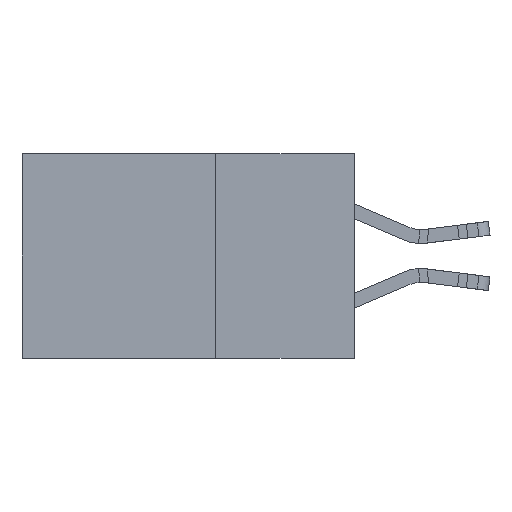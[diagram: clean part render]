
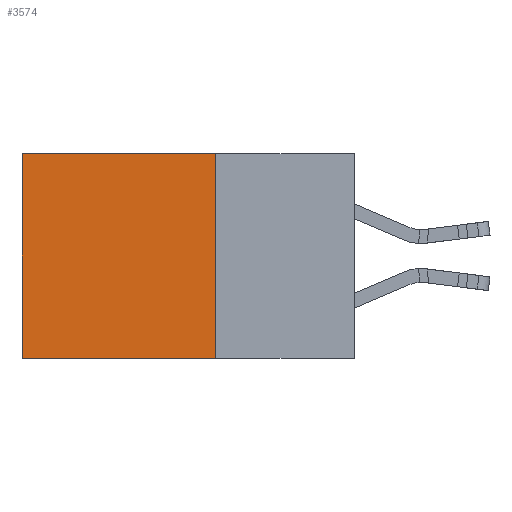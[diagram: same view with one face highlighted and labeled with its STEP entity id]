
A CAD part, left-side view. The second image highlights one B-rep face of the part: STEP entity #3574.
In plain terms, the highlighted planar face has unit normal (-1, 0, 0).
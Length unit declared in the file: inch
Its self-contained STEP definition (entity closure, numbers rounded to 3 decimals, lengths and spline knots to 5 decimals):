
#2606 = DIRECTION ( 'NONE',  ( 0., 0., -1. ) ) ;
#2619 = EDGE_CURVE ( 'NONE', #5461, #28859, #26973, .T. ) ;
#3574 = ADVANCED_FACE ( 'NONE', ( #20780 ), #10908, .F. ) ;
#4157 = ORIENTED_EDGE ( 'NONE', *, *, #2619, .T. ) ;
#5461 = VERTEX_POINT ( 'NONE', #24107 ) ;
#6086 = AXIS2_PLACEMENT_3D ( 'NONE', #10902, #10879, #10489 ) ;
#8408 = CARTESIAN_POINT ( 'NONE',  ( 0.298, 0.25, -0.37 ) ) ;
#8775 = EDGE_LOOP ( 'NONE', ( #9662, #10339, #9751, #4157 ) ) ;
#8953 = CARTESIAN_POINT ( 'NONE',  ( 0.298, 0.6, 0. ) ) ;
#8996 = VERTEX_POINT ( 'NONE', #25405 ) ;
#9223 = VECTOR ( 'NONE', #15777, 39.37008 ) ;
#9247 = VECTOR ( 'NONE', #11238, 39.37008 ) ;
#9662 = ORIENTED_EDGE ( 'NONE', *, *, #21631, .T. ) ;
#9751 = ORIENTED_EDGE ( 'NONE', *, *, #11562, .F. ) ;
#10339 = ORIENTED_EDGE ( 'NONE', *, *, #26287, .F. ) ;
#10489 = DIRECTION ( 'NONE',  ( 0., 0., -1. ) ) ;
#10684 = DIRECTION ( 'NONE',  ( 0., 1., 0. ) ) ;
#10879 = DIRECTION ( 'NONE',  ( 1., 0., 0. ) ) ;
#10902 = CARTESIAN_POINT ( 'NONE',  ( 0.298, 0.25, 0. ) ) ;
#10908 = PLANE ( 'NONE',  #6086 ) ;
#11147 = VECTOR ( 'NONE', #10684, 39.37008 ) ;
#11238 = DIRECTION ( 'NONE',  ( 0., 0., -1. ) ) ;
#11562 = EDGE_CURVE ( 'NONE', #5461, #23902, #22540, .T. ) ;
#12257 = CARTESIAN_POINT ( 'NONE',  ( 0.298, 0.25, 0. ) ) ;
#13918 = CARTESIAN_POINT ( 'NONE',  ( 0.298, 0.25, 0. ) ) ;
#15777 = DIRECTION ( 'NONE',  ( 0., 1., 0. ) ) ;
#20780 = FACE_OUTER_BOUND ( 'NONE', #8775, .T. ) ;
#21631 = EDGE_CURVE ( 'NONE', #28859, #8996, #26994, .T. ) ;
#22540 = LINE ( 'NONE', #13918, #27623 ) ;
#23902 = VERTEX_POINT ( 'NONE', #28627 ) ;
#24107 = CARTESIAN_POINT ( 'NONE',  ( 0.298, 0.25, 0. ) ) ;
#25405 = CARTESIAN_POINT ( 'NONE',  ( 0.298, 0.6, -0.37 ) ) ;
#26287 = EDGE_CURVE ( 'NONE', #23902, #8996, #28810, .T. ) ;
#26973 = LINE ( 'NONE', #12257, #9223 ) ;
#26994 = LINE ( 'NONE', #8953, #9247 ) ;
#27623 = VECTOR ( 'NONE', #2606, 39.37008 ) ;
#28456 = CARTESIAN_POINT ( 'NONE',  ( 0.298, 0.6, 0. ) ) ;
#28627 = CARTESIAN_POINT ( 'NONE',  ( 0.298, 0.25, -0.37 ) ) ;
#28810 = LINE ( 'NONE', #8408, #11147 ) ;
#28859 = VERTEX_POINT ( 'NONE', #28456 ) ;
